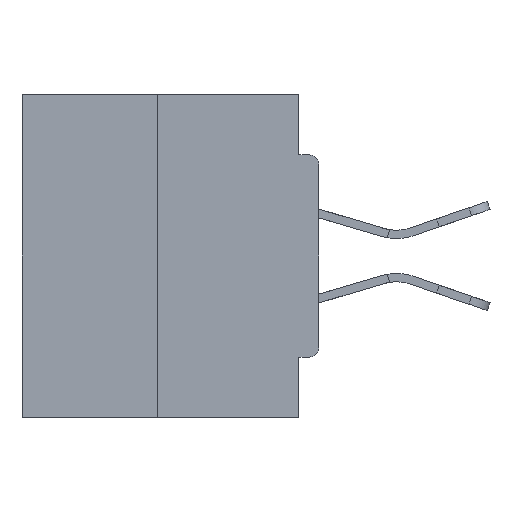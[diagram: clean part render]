
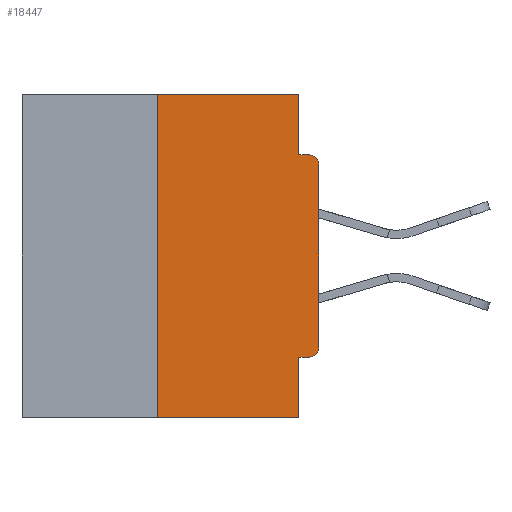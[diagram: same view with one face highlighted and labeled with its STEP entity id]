
A CAD part, left-side view. The second image highlights one B-rep face of the part: STEP entity #18447.
In plain terms, the highlighted planar face has unit normal (-1, 0, 0).
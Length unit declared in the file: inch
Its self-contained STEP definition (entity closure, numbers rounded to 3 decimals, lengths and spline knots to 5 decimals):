
#244 = DIRECTION ( 'NONE',  ( -1., 0., 0. ) ) ;
#1026 = AXIS2_PLACEMENT_3D ( 'NONE', #17179, #244, #14530 ) ;
#1124 = VECTOR ( 'NONE', #29429, 39.37008 ) ;
#2214 = CARTESIAN_POINT ( 'NONE',  ( 0., 0.46, 0. ) ) ;
#2581 = EDGE_CURVE ( 'NONE', #21334, #10267, #28984, .T. ) ;
#2837 = EDGE_CURVE ( 'NONE', #10267, #20173, #17800, .T. ) ;
#3341 = CARTESIAN_POINT ( 'NONE',  ( 0., 0.015, -0.1085 ) ) ;
#4196 = ORIENTED_EDGE ( 'NONE', *, *, #18017, .F. ) ;
#4443 = VECTOR ( 'NONE', #32717, 39.37008 ) ;
#4978 = AXIS2_PLACEMENT_3D ( 'NONE', #3341, #31054, #34823 ) ;
#5038 = ORIENTED_EDGE ( 'NONE', *, *, #19007, .T. ) ;
#7517 = CARTESIAN_POINT ( 'NONE',  ( 0., 0.25, 0. ) ) ;
#7656 = DIRECTION ( 'NONE',  ( 1., 0., 0. ) ) ;
#7993 = LINE ( 'NONE', #17418, #21777 ) ;
#8675 = LINE ( 'NONE', #15088, #1124 ) ;
#9772 = VECTOR ( 'NONE', #10591, 39.37008 ) ;
#10267 = VERTEX_POINT ( 'NONE', #11735 ) ;
#10591 = DIRECTION ( 'NONE',  ( 0., 0., 1. ) ) ;
#10753 = PLANE ( 'NONE',  #27584 ) ;
#11040 = DIRECTION ( 'NONE',  ( 0., -1., 0. ) ) ;
#11218 = CARTESIAN_POINT ( 'NONE',  ( 0., 0., -0.3915 ) ) ;
#11561 = VERTEX_POINT ( 'NONE', #30797 ) ;
#11735 = CARTESIAN_POINT ( 'NONE',  ( 0., 0.031, -0.4065 ) ) ;
#11754 = CARTESIAN_POINT ( 'NONE',  ( 0., 0.031, -0.0935 ) ) ;
#12412 = DIRECTION ( 'NONE',  ( 0., 0., -1. ) ) ;
#12820 = ORIENTED_EDGE ( 'NONE', *, *, #32933, .T. ) ;
#12914 = VERTEX_POINT ( 'NONE', #11218 ) ;
#13055 = CIRCLE ( 'NONE', #1026, 0.015 ) ;
#13090 = CARTESIAN_POINT ( 'NONE',  ( 0., 0.25, 0. ) ) ;
#13814 = VECTOR ( 'NONE', #25603, 39.37008 ) ;
#14378 = ORIENTED_EDGE ( 'NONE', *, *, #32817, .F. ) ;
#14396 = ORIENTED_EDGE ( 'NONE', *, *, #17443, .F. ) ;
#14530 = DIRECTION ( 'NONE',  ( 0., 0., -1. ) ) ;
#14659 = VECTOR ( 'NONE', #12412, 39.37008 ) ;
#14665 = VERTEX_POINT ( 'NONE', #11754 ) ;
#14892 = DIRECTION ( 'NONE',  ( 0., -1., 0. ) ) ;
#15088 = CARTESIAN_POINT ( 'NONE',  ( 0., 0., 0. ) ) ;
#15488 = CARTESIAN_POINT ( 'NONE',  ( 0., 0.46, 0. ) ) ;
#15582 = CARTESIAN_POINT ( 'NONE',  ( 0., 0.031, -0.5 ) ) ;
#16533 = CARTESIAN_POINT ( 'NONE',  ( 0., 0.46, -0.5 ) ) ;
#16856 = LINE ( 'NONE', #23496, #14659 ) ;
#16922 = VECTOR ( 'NONE', #18349, 39.37008 ) ;
#17179 = CARTESIAN_POINT ( 'NONE',  ( 0., 0.015, -0.3915 ) ) ;
#17330 = FACE_OUTER_BOUND ( 'NONE', #29390, .T. ) ;
#17418 = CARTESIAN_POINT ( 'NONE',  ( 0., 0., -0.0935 ) ) ;
#17443 = EDGE_CURVE ( 'NONE', #11561, #14665, #16856, .T. ) ;
#17800 = LINE ( 'NONE', #15582, #16922 ) ;
#18017 = EDGE_CURVE ( 'NONE', #22724, #11561, #28448, .T. ) ;
#18349 = DIRECTION ( 'NONE',  ( 0., 0., -1. ) ) ;
#18447 = ADVANCED_FACE ( 'NONE', ( #17330 ), #10753, .F. ) ;
#18764 = CARTESIAN_POINT ( 'NONE',  ( 0., 0., -0.4065 ) ) ;
#19007 = EDGE_CURVE ( 'NONE', #20890, #20991, #23025, .T. ) ;
#19436 = EDGE_CURVE ( 'NONE', #14665, #20991, #7993, .T. ) ;
#20173 = VERTEX_POINT ( 'NONE', #24527 ) ;
#20633 = CARTESIAN_POINT ( 'NONE',  ( 0., 0.015, -0.0935 ) ) ;
#20890 = VERTEX_POINT ( 'NONE', #34846 ) ;
#20991 = VERTEX_POINT ( 'NONE', #20633 ) ;
#21320 = LINE ( 'NONE', #13090, #9772 ) ;
#21334 = VERTEX_POINT ( 'NONE', #34715 ) ;
#21698 = DIRECTION ( 'NONE',  ( 0., 0., -1. ) ) ;
#21777 = VECTOR ( 'NONE', #14892, 39.37008 ) ;
#22724 = VERTEX_POINT ( 'NONE', #7517 ) ;
#23025 = CIRCLE ( 'NONE', #4978, 0.015 ) ;
#23318 = EDGE_CURVE ( 'NONE', #21334, #12914, #13055, .T. ) ;
#23496 = CARTESIAN_POINT ( 'NONE',  ( 0., 0.031, 0. ) ) ;
#24527 = CARTESIAN_POINT ( 'NONE',  ( 0., 0.031, -0.5 ) ) ;
#25603 = DIRECTION ( 'NONE',  ( 0., 1., 0. ) ) ;
#25814 = LINE ( 'NONE', #16533, #34733 ) ;
#26486 = CARTESIAN_POINT ( 'NONE',  ( 0., 0.25, -0.5 ) ) ;
#26791 = VERTEX_POINT ( 'NONE', #26486 ) ;
#27584 = AXIS2_PLACEMENT_3D ( 'NONE', #2214, #7656, #21698 ) ;
#28448 = LINE ( 'NONE', #15488, #4443 ) ;
#28984 = LINE ( 'NONE', #18764, #13814 ) ;
#29390 = EDGE_LOOP ( 'NONE', ( #4196, #14378, #12820, #34580, #33963, #36911, #30859, #5038, #33446, #14396 ) ) ;
#29429 = DIRECTION ( 'NONE',  ( 0., 0., 1. ) ) ;
#30797 = CARTESIAN_POINT ( 'NONE',  ( 0., 0.031, 0. ) ) ;
#30859 = ORIENTED_EDGE ( 'NONE', *, *, #35545, .T. ) ;
#31054 = DIRECTION ( 'NONE',  ( -1., 0., 0. ) ) ;
#32717 = DIRECTION ( 'NONE',  ( 0., -1., 0. ) ) ;
#32817 = EDGE_CURVE ( 'NONE', #26791, #22724, #21320, .T. ) ;
#32933 = EDGE_CURVE ( 'NONE', #26791, #20173, #25814, .T. ) ;
#33446 = ORIENTED_EDGE ( 'NONE', *, *, #19436, .F. ) ;
#33963 = ORIENTED_EDGE ( 'NONE', *, *, #2581, .F. ) ;
#34580 = ORIENTED_EDGE ( 'NONE', *, *, #2837, .F. ) ;
#34715 = CARTESIAN_POINT ( 'NONE',  ( 0., 0.015, -0.4065 ) ) ;
#34733 = VECTOR ( 'NONE', #11040, 39.37008 ) ;
#34823 = DIRECTION ( 'NONE',  ( 0., 0., -1. ) ) ;
#34846 = CARTESIAN_POINT ( 'NONE',  ( 0., 0., -0.1085 ) ) ;
#35545 = EDGE_CURVE ( 'NONE', #12914, #20890, #8675, .T. ) ;
#36911 = ORIENTED_EDGE ( 'NONE', *, *, #23318, .T. ) ;
